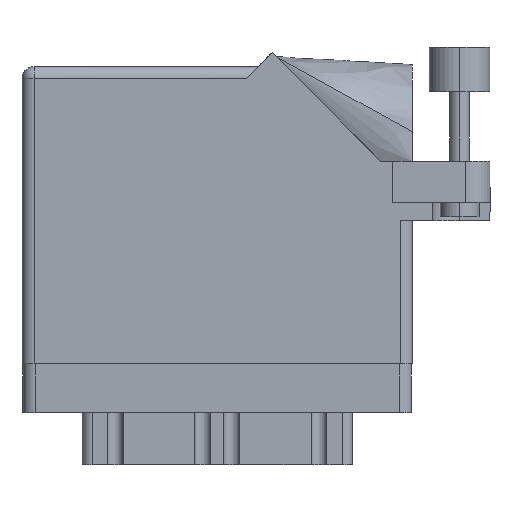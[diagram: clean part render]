
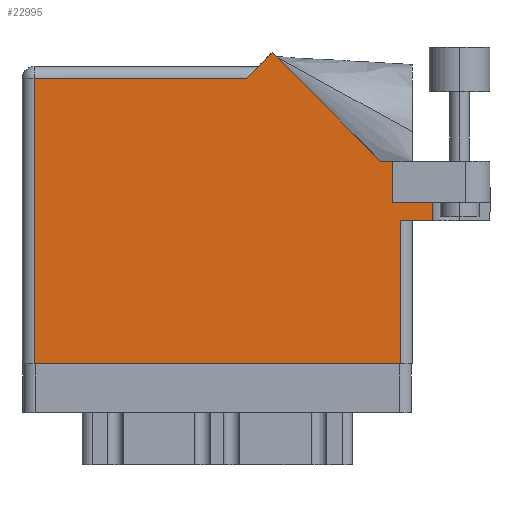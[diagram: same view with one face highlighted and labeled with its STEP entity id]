
A CAD part, front view. The second image highlights one B-rep face of the part: STEP entity #22995.
In plain terms, the highlighted face is planar.
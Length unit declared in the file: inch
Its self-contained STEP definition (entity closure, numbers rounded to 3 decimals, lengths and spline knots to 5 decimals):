
#1473 = EDGE_CURVE ( 'NONE', #16094, #24129, #23481, .T. ) ;
#1962 = LINE ( 'NONE', #31872, #14077 ) ;
#2436 = LINE ( 'NONE', #13234, #2690 ) ;
#2690 = VECTOR ( 'NONE', #34826, 39.37008 ) ;
#4318 = VERTEX_POINT ( 'NONE', #10472 ) ;
#4373 = ORIENTED_EDGE ( 'NONE', *, *, #27264, .T. ) ;
#4765 = VECTOR ( 'NONE', #32904, 39.37008 ) ;
#5052 = CARTESIAN_POINT ( 'NONE',  ( 1.91, 0.831, 0. ) ) ;
#5356 = EDGE_CURVE ( 'NONE', #34151, #4318, #2436, .T. ) ;
#5646 = FACE_OUTER_BOUND ( 'NONE', #6296, .T. ) ;
#6035 = DIRECTION ( 'NONE',  ( 0., 1., 0. ) ) ;
#6296 = EDGE_LOOP ( 'NONE', ( #9929, #13431, #18081, #21709, #25468, #9695, #20700, #17319, #18109, #4373, #24457 ) ) ;
#6493 = DIRECTION ( 'NONE',  ( 0., -1., 0. ) ) ;
#7174 = VERTEX_POINT ( 'NONE', #16307 ) ;
#7830 = DIRECTION ( 'NONE',  ( 0., 0., -1. ) ) ;
#7917 = LINE ( 'NONE', #34655, #16338 ) ;
#8484 = PLANE ( 'NONE',  #21465 ) ;
#8704 = CARTESIAN_POINT ( 'NONE',  ( 1.948, 0.737, 0. ) ) ;
#8937 = VERTEX_POINT ( 'NONE', #16683 ) ;
#8959 = CARTESIAN_POINT ( 'NONE',  ( 1.91, 0.831, 0. ) ) ;
#9298 = EDGE_CURVE ( 'NONE', #31172, #4318, #27928, .T. ) ;
#9695 = ORIENTED_EDGE ( 'NONE', *, *, #1473, .T. ) ;
#9929 = ORIENTED_EDGE ( 'NONE', *, *, #22060, .T. ) ;
#10472 = CARTESIAN_POINT ( 'NONE',  ( 2.1115, 0.737, 0. ) ) ;
#10796 = CARTESIAN_POINT ( 'NONE',  ( 0.062, 1.468, 0. ) ) ;
#11999 = VERTEX_POINT ( 'NONE', #21303 ) ;
#12305 = EDGE_CURVE ( 'NONE', #31423, #7174, #29236, .T. ) ;
#13036 = VECTOR ( 'NONE', #22345, 39.37008 ) ;
#13234 = CARTESIAN_POINT ( 'NONE',  ( 2.01, 0.737, 0. ) ) ;
#13431 = ORIENTED_EDGE ( 'NONE', *, *, #26360, .T. ) ;
#14077 = VECTOR ( 'NONE', #18247, 39.37008 ) ;
#14434 = CARTESIAN_POINT ( 'NONE',  ( 1.91, 0.831, 0. ) ) ;
#15827 = LINE ( 'NONE', #33898, #20571 ) ;
#16094 = VERTEX_POINT ( 'NONE', #14434 ) ;
#16307 = CARTESIAN_POINT ( 'NONE',  ( 1.155, 1.468, 0. ) ) ;
#16338 = VECTOR ( 'NONE', #18537, 39.37008 ) ;
#16620 = DIRECTION ( 'NONE',  ( -1., 0., 0. ) ) ;
#16683 = CARTESIAN_POINT ( 'NONE',  ( 0.062, 0., 0. ) ) ;
#17108 = DIRECTION ( 'NONE',  ( 1., 0., 0. ) ) ;
#17309 = CARTESIAN_POINT ( 'NONE',  ( 1.948, 0.737, 0. ) ) ;
#17319 = ORIENTED_EDGE ( 'NONE', *, *, #26649, .T. ) ;
#18081 = ORIENTED_EDGE ( 'NONE', *, *, #5356, .T. ) ;
#18109 = ORIENTED_EDGE ( 'NONE', *, *, #12305, .T. ) ;
#18133 = DIRECTION ( 'NONE',  ( -1., 0., 0. ) ) ;
#18195 = CARTESIAN_POINT ( 'NONE',  ( 2.1115, 0.831, 0. ) ) ;
#18247 = DIRECTION ( 'NONE',  ( -0.707, 0.707, 0. ) ) ;
#18537 = DIRECTION ( 'NONE',  ( 1., 0., 0. ) ) ;
#18605 = EDGE_CURVE ( 'NONE', #32225, #8937, #24241, .T. ) ;
#19149 = LINE ( 'NONE', #8704, #24781 ) ;
#19507 = CARTESIAN_POINT ( 'NONE',  ( 2.41, 1.044, 0. ) ) ;
#20571 = VECTOR ( 'NONE', #18133, 39.37008 ) ;
#20700 = ORIENTED_EDGE ( 'NONE', *, *, #33228, .T. ) ;
#20817 = DIRECTION ( 'NONE',  ( 0., 1., 0. ) ) ;
#20921 = VERTEX_POINT ( 'NONE', #27732 ) ;
#21303 = CARTESIAN_POINT ( 'NONE',  ( 1.84442, 1.044, 0. ) ) ;
#21465 = AXIS2_PLACEMENT_3D ( 'NONE', #31908, #7830, #16620 ) ;
#21709 = ORIENTED_EDGE ( 'NONE', *, *, #9298, .F. ) ;
#22060 = EDGE_CURVE ( 'NONE', #8937, #20921, #7917, .T. ) ;
#22229 = LINE ( 'NONE', #8959, #28083 ) ;
#22345 = DIRECTION ( 'NONE',  ( -1., 0., 0. ) ) ;
#22995 = ADVANCED_FACE ( 'NONE', ( #5646 ), #8484, .F. ) ;
#23481 = LINE ( 'NONE', #5052, #28973 ) ;
#23585 = CARTESIAN_POINT ( 'NONE',  ( 1.217, 1.53, 0. ) ) ;
#24129 = VERTEX_POINT ( 'NONE', #31299 ) ;
#24241 = LINE ( 'NONE', #24759, #4765 ) ;
#24359 = EDGE_CURVE ( 'NONE', #16094, #31172, #22229, .T. ) ;
#24457 = ORIENTED_EDGE ( 'NONE', *, *, #18605, .T. ) ;
#24759 = CARTESIAN_POINT ( 'NONE',  ( 0.062, 0., 0. ) ) ;
#24781 = VECTOR ( 'NONE', #6035, 39.37008 ) ;
#25468 = ORIENTED_EDGE ( 'NONE', *, *, #24359, .F. ) ;
#26360 = EDGE_CURVE ( 'NONE', #20921, #34151, #19149, .T. ) ;
#26649 = EDGE_CURVE ( 'NONE', #11999, #31423, #1962, .T. ) ;
#27264 = EDGE_CURVE ( 'NONE', #7174, #32225, #15827, .T. ) ;
#27487 = LINE ( 'NONE', #19507, #13036 ) ;
#27732 = CARTESIAN_POINT ( 'NONE',  ( 1.948, 0., 0. ) ) ;
#27928 = LINE ( 'NONE', #33232, #29437 ) ;
#28083 = VECTOR ( 'NONE', #17108, 39.37008 ) ;
#28973 = VECTOR ( 'NONE', #20817, 39.37008 ) ;
#29236 = LINE ( 'NONE', #23585, #32612 ) ;
#29303 = CARTESIAN_POINT ( 'NONE',  ( 1.28771, 1.60071, 0. ) ) ;
#29437 = VECTOR ( 'NONE', #6493, 39.37008 ) ;
#31172 = VERTEX_POINT ( 'NONE', #18195 ) ;
#31299 = CARTESIAN_POINT ( 'NONE',  ( 1.91, 1.044, 0. ) ) ;
#31423 = VERTEX_POINT ( 'NONE', #29303 ) ;
#31549 = DIRECTION ( 'NONE',  ( -0.707, -0.707, 0. ) ) ;
#31872 = CARTESIAN_POINT ( 'NONE',  ( 1.84442, 1.044, 0. ) ) ;
#31908 = CARTESIAN_POINT ( 'NONE',  ( 0., 1.53, 0. ) ) ;
#32225 = VERTEX_POINT ( 'NONE', #10796 ) ;
#32612 = VECTOR ( 'NONE', #31549, 39.37008 ) ;
#32904 = DIRECTION ( 'NONE',  ( 0., -1., 0. ) ) ;
#33228 = EDGE_CURVE ( 'NONE', #24129, #11999, #27487, .T. ) ;
#33232 = CARTESIAN_POINT ( 'NONE',  ( 2.1115, 1.16177, 0. ) ) ;
#33898 = CARTESIAN_POINT ( 'NONE',  ( 0., 1.468, 0. ) ) ;
#34151 = VERTEX_POINT ( 'NONE', #17309 ) ;
#34655 = CARTESIAN_POINT ( 'NONE',  ( 0., 0., 0. ) ) ;
#34826 = DIRECTION ( 'NONE',  ( 1., 0., 0. ) ) ;
